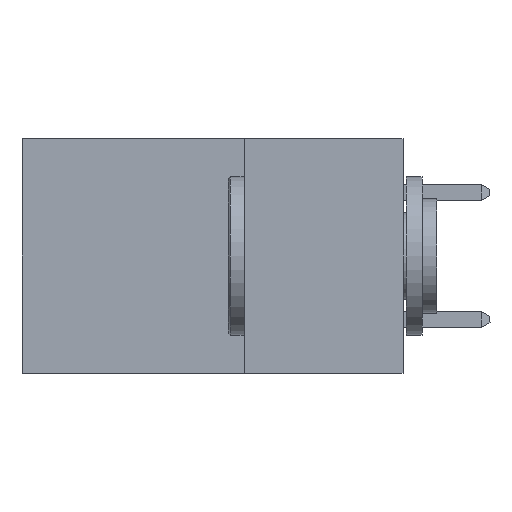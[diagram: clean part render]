
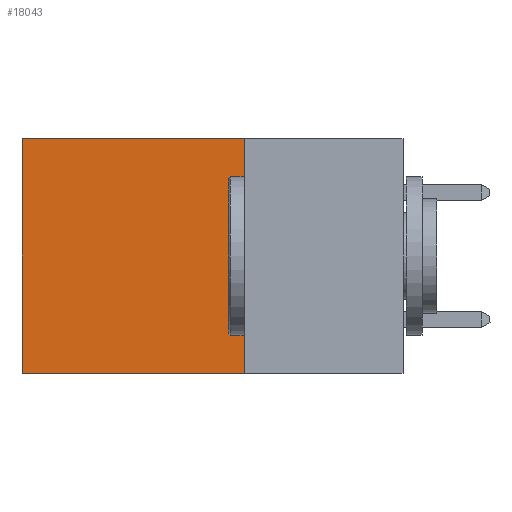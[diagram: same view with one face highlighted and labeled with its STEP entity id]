
A CAD part, left-side view. The second image highlights one B-rep face of the part: STEP entity #18043.
In plain terms, the highlighted planar face has unit normal (-1, 0, 0).
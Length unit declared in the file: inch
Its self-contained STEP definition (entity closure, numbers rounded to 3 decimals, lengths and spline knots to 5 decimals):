
#444 = CARTESIAN_POINT ( 'NONE',  ( 0.2875, 0.6, 0. ) ) ;
#685 = CARTESIAN_POINT ( 'NONE',  ( 0.2875, 0.25, 0. ) ) ;
#1029 = DIRECTION ( 'NONE',  ( 0., 0., -1. ) ) ;
#1408 = ORIENTED_EDGE ( 'NONE', *, *, #14578, .F. ) ;
#2206 = LINE ( 'NONE', #685, #9928 ) ;
#2265 = DIRECTION ( 'NONE',  ( 0., 1., 0. ) ) ;
#2317 = LINE ( 'NONE', #444, #14691 ) ;
#5288 = CARTESIAN_POINT ( 'NONE',  ( 0.2875, 0.25, -0.37 ) ) ;
#5610 = CARTESIAN_POINT ( 'NONE',  ( 0.2875, 0.25, 0. ) ) ;
#5810 = LINE ( 'NONE', #5288, #13626 ) ;
#6828 = DIRECTION ( 'NONE',  ( 0., 1., 0. ) ) ;
#7096 = CARTESIAN_POINT ( 'NONE',  ( 0.2875, 0.25, 0. ) ) ;
#7202 = VERTEX_POINT ( 'NONE', #8168 ) ;
#7934 = ORIENTED_EDGE ( 'NONE', *, *, #17903, .F. ) ;
#8168 = CARTESIAN_POINT ( 'NONE',  ( 0.2875, 0.25, 0. ) ) ;
#8476 = EDGE_CURVE ( 'NONE', #17287, #12600, #2317, .T. ) ;
#8592 = CARTESIAN_POINT ( 'NONE',  ( 0.2875, 0.6, 0. ) ) ;
#8705 = CARTESIAN_POINT ( 'NONE',  ( 0.2875, 0.6, -0.37 ) ) ;
#9928 = VECTOR ( 'NONE', #2265, 39.37008 ) ;
#10316 = DIRECTION ( 'NONE',  ( 1., 0., 0. ) ) ;
#11067 = VECTOR ( 'NONE', #16473, 39.37008 ) ;
#11250 = EDGE_CURVE ( 'NONE', #7202, #17287, #2206, .T. ) ;
#11576 = LINE ( 'NONE', #5610, #11067 ) ;
#12600 = VERTEX_POINT ( 'NONE', #8705 ) ;
#13626 = VECTOR ( 'NONE', #6828, 39.37008 ) ;
#14578 = EDGE_CURVE ( 'NONE', #7202, #15711, #11576, .T. ) ;
#14691 = VECTOR ( 'NONE', #15916, 39.37008 ) ;
#15326 = FACE_OUTER_BOUND ( 'NONE', #19710, .T. ) ;
#15711 = VERTEX_POINT ( 'NONE', #18554 ) ;
#15916 = DIRECTION ( 'NONE',  ( 0., 0., -1. ) ) ;
#16473 = DIRECTION ( 'NONE',  ( 0., 0., -1. ) ) ;
#17287 = VERTEX_POINT ( 'NONE', #8592 ) ;
#17745 = ORIENTED_EDGE ( 'NONE', *, *, #8476, .T. ) ;
#17903 = EDGE_CURVE ( 'NONE', #15711, #12600, #5810, .T. ) ;
#18043 = ADVANCED_FACE ( 'NONE', ( #15326 ), #19532, .F. ) ;
#18554 = CARTESIAN_POINT ( 'NONE',  ( 0.2875, 0.25, -0.37 ) ) ;
#18584 = ORIENTED_EDGE ( 'NONE', *, *, #11250, .T. ) ;
#19021 = AXIS2_PLACEMENT_3D ( 'NONE', #7096, #10316, #1029 ) ;
#19532 = PLANE ( 'NONE',  #19021 ) ;
#19710 = EDGE_LOOP ( 'NONE', ( #17745, #7934, #1408, #18584 ) ) ;
